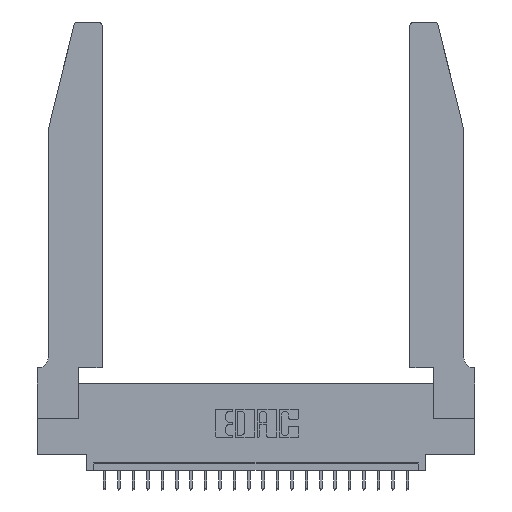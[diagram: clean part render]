
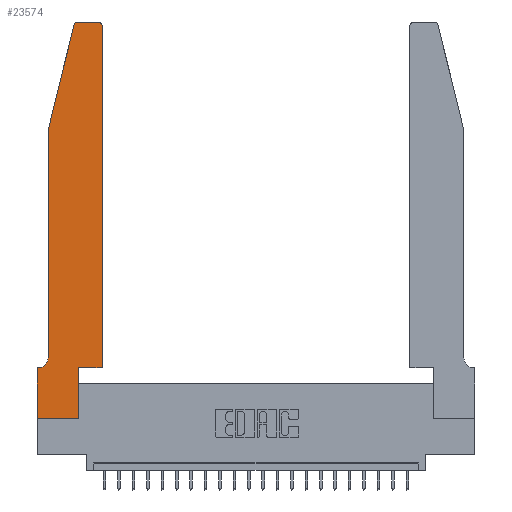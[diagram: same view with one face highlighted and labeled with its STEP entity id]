
A CAD part, top view. The second image highlights one B-rep face of the part: STEP entity #23574.
In plain terms, the highlighted planar face has unit normal (0, 0, 1).
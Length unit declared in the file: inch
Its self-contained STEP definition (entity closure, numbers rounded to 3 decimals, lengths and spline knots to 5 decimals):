
#55 = ORIENTED_EDGE ( 'NONE', *, *, #11408, .T. ) ;
#196 = VERTEX_POINT ( 'NONE', #18630 ) ;
#533 = ORIENTED_EDGE ( 'NONE', *, *, #15065, .T. ) ;
#696 = LINE ( 'NONE', #15811, #2598 ) ;
#1002 = EDGE_CURVE ( 'NONE', #3508, #8109, #15591, .T. ) ;
#1030 = CARTESIAN_POINT ( 'NONE',  ( 0.0755, 2., 0.37 ) ) ;
#1059 = ORIENTED_EDGE ( 'NONE', *, *, #4736, .T. ) ;
#1420 = LINE ( 'NONE', #10489, #14884 ) ;
#2598 = VECTOR ( 'NONE', #15930, 39.37008 ) ;
#2993 = DIRECTION ( 'NONE',  ( 0., 0., 1. ) ) ;
#3504 = VECTOR ( 'NONE', #14059, 39.37008 ) ;
#3508 = VERTEX_POINT ( 'NONE', #22718 ) ;
#3535 = VERTEX_POINT ( 'NONE', #20887 ) ;
#3580 = EDGE_LOOP ( 'NONE', ( #15106, #1059, #19735, #10396, #8805, #20001, #15556, #18771, #533, #20857, #55, #9801 ) ) ;
#3696 = VECTOR ( 'NONE', #23369, 39.37008 ) ;
#4098 = DIRECTION ( 'NONE',  ( 0., 1., 0. ) ) ;
#4199 = CIRCLE ( 'NONE', #5766, 0.03 ) ;
#4703 = LINE ( 'NONE', #1030, #12319 ) ;
#4736 = EDGE_CURVE ( 'NONE', #8109, #196, #16482, .T. ) ;
#5320 = DIRECTION ( 'NONE',  ( 1., 0., 0. ) ) ;
#5766 = AXIS2_PLACEMENT_3D ( 'NONE', #21503, #2993, #8493 ) ;
#5882 = DIRECTION ( 'NONE',  ( 1., 0., 0. ) ) ;
#6206 = VERTEX_POINT ( 'NONE', #10122 ) ;
#6310 = EDGE_CURVE ( 'NONE', #6206, #11203, #16417, .T. ) ;
#6435 = LINE ( 'NONE', #13943, #18089 ) ;
#6560 = CARTESIAN_POINT ( 'NONE',  ( 0., 0., 0.37 ) ) ;
#6728 = VERTEX_POINT ( 'NONE', #12980 ) ;
#6826 = CARTESIAN_POINT ( 'NONE',  ( 0.4505, 0.35, 0.37 ) ) ;
#6854 = EDGE_CURVE ( 'NONE', #23805, #15332, #20182, .T. ) ;
#7173 = PLANE ( 'NONE',  #12813 ) ;
#7718 = DIRECTION ( 'NONE',  ( 0., 1., 0. ) ) ;
#8109 = VERTEX_POINT ( 'NONE', #11617 ) ;
#8192 = CARTESIAN_POINT ( 'NONE',  ( 0.2865, 0.35, 0.37 ) ) ;
#8486 = DIRECTION ( 'NONE',  ( -0.239, -0.971, 0. ) ) ;
#8493 = DIRECTION ( 'NONE',  ( 1., 0., 0. ) ) ;
#8805 = ORIENTED_EDGE ( 'NONE', *, *, #6310, .T. ) ;
#9088 = LINE ( 'NONE', #15261, #20256 ) ;
#9669 = DIRECTION ( 'NONE',  ( 0., 0., 1. ) ) ;
#9801 = ORIENTED_EDGE ( 'NONE', *, *, #23655, .T. ) ;
#10122 = CARTESIAN_POINT ( 'NONE',  ( 0.0755, 0.42, 0.37 ) ) ;
#10396 = ORIENTED_EDGE ( 'NONE', *, *, #11058, .T. ) ;
#10454 = EDGE_CURVE ( 'NONE', #196, #6728, #4703, .T. ) ;
#10489 = CARTESIAN_POINT ( 'NONE',  ( 0.4505, 0.35, 0.37 ) ) ;
#11058 = EDGE_CURVE ( 'NONE', #6728, #6206, #21225, .T. ) ;
#11203 = VERTEX_POINT ( 'NONE', #20584 ) ;
#11371 = CARTESIAN_POINT ( 'NONE',  ( 0., 0.35, 0.37 ) ) ;
#11408 = EDGE_CURVE ( 'NONE', #14393, #3535, #13056, .T. ) ;
#11586 = CARTESIAN_POINT ( 'NONE',  ( 0.4505, 0.35, 0.37 ) ) ;
#11617 = CARTESIAN_POINT ( 'NONE',  ( 0.284, 2.75, 0.37 ) ) ;
#12270 = EDGE_CURVE ( 'NONE', #20990, #23805, #696, .T. ) ;
#12319 = VECTOR ( 'NONE', #8486, 39.37008 ) ;
#12813 = AXIS2_PLACEMENT_3D ( 'NONE', #22385, #22129, #5320 ) ;
#12980 = CARTESIAN_POINT ( 'NONE',  ( 0.0755, 2., 0.37 ) ) ;
#13056 = LINE ( 'NONE', #11586, #15126 ) ;
#13497 = CARTESIAN_POINT ( 'NONE',  ( 0.0755, 2., 0.37 ) ) ;
#13609 = CARTESIAN_POINT ( 'NONE',  ( 0.2865, 0., 0.37 ) ) ;
#13943 = CARTESIAN_POINT ( 'NONE',  ( 0.0755, 0.35, 0.37 ) ) ;
#14059 = DIRECTION ( 'NONE',  ( 1., 0., 0. ) ) ;
#14393 = VERTEX_POINT ( 'NONE', #6826 ) ;
#14884 = VECTOR ( 'NONE', #16178, 39.37008 ) ;
#15065 = EDGE_CURVE ( 'NONE', #15332, #18471, #9088, .T. ) ;
#15106 = ORIENTED_EDGE ( 'NONE', *, *, #1002, .T. ) ;
#15126 = VECTOR ( 'NONE', #4098, 39.37008 ) ;
#15261 = CARTESIAN_POINT ( 'NONE',  ( 0.2865, 0.35, 0.37 ) ) ;
#15332 = VERTEX_POINT ( 'NONE', #13609 ) ;
#15556 = ORIENTED_EDGE ( 'NONE', *, *, #12270, .T. ) ;
#15591 = LINE ( 'NONE', #17532, #3696 ) ;
#15811 = CARTESIAN_POINT ( 'NONE',  ( 0., 0., 0.37 ) ) ;
#15930 = DIRECTION ( 'NONE',  ( 0., -1., 0. ) ) ;
#16159 = CARTESIAN_POINT ( 'NONE',  ( 0.0055, 0.42, 0.37 ) ) ;
#16178 = DIRECTION ( 'NONE',  ( 1., 0., 0. ) ) ;
#16417 = CIRCLE ( 'NONE', #20710, 0.07 ) ;
#16482 = CIRCLE ( 'NONE', #19978, 0.03 ) ;
#17532 = CARTESIAN_POINT ( 'NONE',  ( 0.2605, 2.75, 0.37 ) ) ;
#17615 = EDGE_CURVE ( 'NONE', #18471, #14393, #1420, .T. ) ;
#18089 = VECTOR ( 'NONE', #21395, 39.37008 ) ;
#18471 = VERTEX_POINT ( 'NONE', #8192 ) ;
#18630 = CARTESIAN_POINT ( 'NONE',  ( 0.25487, 2.72718, 0.37 ) ) ;
#18771 = ORIENTED_EDGE ( 'NONE', *, *, #6854, .T. ) ;
#19022 = CARTESIAN_POINT ( 'NONE',  ( 0.284, 2.72, 0.37 ) ) ;
#19735 = ORIENTED_EDGE ( 'NONE', *, *, #10454, .T. ) ;
#19924 = DIRECTION ( 'NONE',  ( -1., 0., 0. ) ) ;
#19925 = EDGE_CURVE ( 'NONE', #11203, #20990, #6435, .T. ) ;
#19978 = AXIS2_PLACEMENT_3D ( 'NONE', #19022, #9669, #5882 ) ;
#20001 = ORIENTED_EDGE ( 'NONE', *, *, #19925, .T. ) ;
#20182 = LINE ( 'NONE', #6560, #3504 ) ;
#20256 = VECTOR ( 'NONE', #7718, 39.37008 ) ;
#20584 = CARTESIAN_POINT ( 'NONE',  ( 0.0055, 0.35, 0.37 ) ) ;
#20710 = AXIS2_PLACEMENT_3D ( 'NONE', #16159, #23583, #19924 ) ;
#20857 = ORIENTED_EDGE ( 'NONE', *, *, #17615, .T. ) ;
#20887 = CARTESIAN_POINT ( 'NONE',  ( 0.4505, 2.72, 0.37 ) ) ;
#20978 = DIRECTION ( 'NONE',  ( 0., -1., 0. ) ) ;
#20990 = VERTEX_POINT ( 'NONE', #11371 ) ;
#21225 = LINE ( 'NONE', #13497, #21729 ) ;
#21395 = DIRECTION ( 'NONE',  ( -1., 0., 0. ) ) ;
#21503 = CARTESIAN_POINT ( 'NONE',  ( 0.4205, 2.72, 0.37 ) ) ;
#21729 = VECTOR ( 'NONE', #20978, 39.37008 ) ;
#22129 = DIRECTION ( 'NONE',  ( 0., 0., 1. ) ) ;
#22385 = CARTESIAN_POINT ( 'NONE',  ( 0., 0.35, 0.37 ) ) ;
#22718 = CARTESIAN_POINT ( 'NONE',  ( 0.4205, 2.75, 0.37 ) ) ;
#22732 = CARTESIAN_POINT ( 'NONE',  ( 0., 0., 0.37 ) ) ;
#23369 = DIRECTION ( 'NONE',  ( -1., 0., 0. ) ) ;
#23574 = ADVANCED_FACE ( 'NONE', ( #23959 ), #7173, .T. ) ;
#23583 = DIRECTION ( 'NONE',  ( 0., 0., -1. ) ) ;
#23655 = EDGE_CURVE ( 'NONE', #3535, #3508, #4199, .T. ) ;
#23805 = VERTEX_POINT ( 'NONE', #22732 ) ;
#23959 = FACE_OUTER_BOUND ( 'NONE', #3580, .T. ) ;
